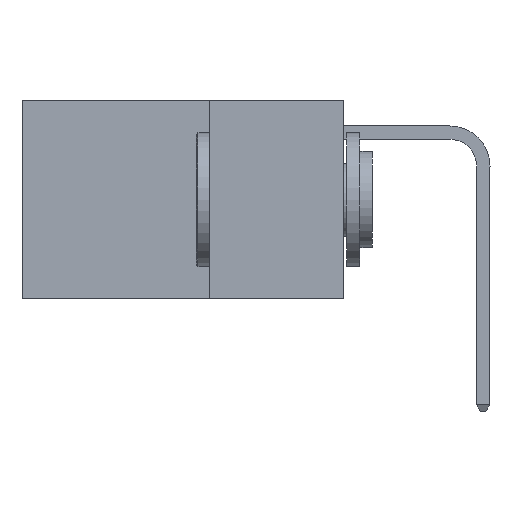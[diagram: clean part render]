
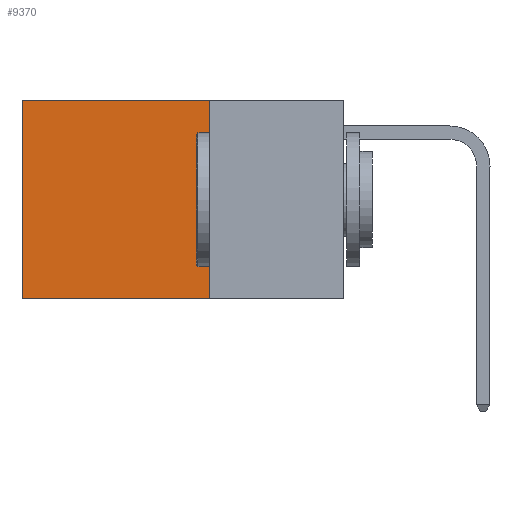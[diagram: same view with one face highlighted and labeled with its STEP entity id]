
A CAD part, left-side view. The second image highlights one B-rep face of the part: STEP entity #9370.
In plain terms, the highlighted planar face has unit normal (-1, 0, 0).
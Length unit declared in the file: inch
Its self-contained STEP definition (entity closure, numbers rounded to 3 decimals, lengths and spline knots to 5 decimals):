
#514 = EDGE_LOOP ( 'NONE', ( #15998, #1596, #9890, #17307 ) ) ;
#658 = CARTESIAN_POINT ( 'NONE',  ( 0.2625, 0.25, 0. ) ) ;
#696 = DIRECTION ( 'NONE',  ( 0., 0., -1. ) ) ;
#1596 = ORIENTED_EDGE ( 'NONE', *, *, #17029, .F. ) ;
#2420 = LINE ( 'NONE', #6323, #17493 ) ;
#3507 = DIRECTION ( 'NONE',  ( 0., 0., -1. ) ) ;
#3826 = VERTEX_POINT ( 'NONE', #658 ) ;
#3992 = VERTEX_POINT ( 'NONE', #5757 ) ;
#4047 = LINE ( 'NONE', #18514, #5840 ) ;
#4448 = EDGE_CURVE ( 'NONE', #9335, #3992, #13016, .T. ) ;
#4850 = EDGE_CURVE ( 'NONE', #3826, #9335, #2420, .T. ) ;
#5757 = CARTESIAN_POINT ( 'NONE',  ( 0.2625, 0.6, -0.37 ) ) ;
#5840 = VECTOR ( 'NONE', #3507, 39.37008 ) ;
#5875 = DIRECTION ( 'NONE',  ( 0., 0., -1. ) ) ;
#5886 = CARTESIAN_POINT ( 'NONE',  ( 0.2625, 0.6, 0. ) ) ;
#6323 = CARTESIAN_POINT ( 'NONE',  ( 0.2625, 0.25, 0. ) ) ;
#6891 = CARTESIAN_POINT ( 'NONE',  ( 0.2625, 0.25, -0.37 ) ) ;
#7074 = CARTESIAN_POINT ( 'NONE',  ( 0.2625, 0.25, -0.37 ) ) ;
#8128 = CARTESIAN_POINT ( 'NONE',  ( 0.2625, 0.6, 0. ) ) ;
#9335 = VERTEX_POINT ( 'NONE', #8128 ) ;
#9370 = ADVANCED_FACE ( 'NONE', ( #18680 ), #11130, .F. ) ;
#9466 = VECTOR ( 'NONE', #5875, 39.37008 ) ;
#9693 = DIRECTION ( 'NONE',  ( 1., 0., 0. ) ) ;
#9890 = ORIENTED_EDGE ( 'NONE', *, *, #16073, .F. ) ;
#10082 = VECTOR ( 'NONE', #19084, 39.37008 ) ;
#11130 = PLANE ( 'NONE',  #11276 ) ;
#11276 = AXIS2_PLACEMENT_3D ( 'NONE', #17231, #9693, #696 ) ;
#13016 = LINE ( 'NONE', #5886, #9466 ) ;
#13539 = DIRECTION ( 'NONE',  ( 0., 1., 0. ) ) ;
#14133 = LINE ( 'NONE', #7074, #10082 ) ;
#15998 = ORIENTED_EDGE ( 'NONE', *, *, #4448, .T. ) ;
#16073 = EDGE_CURVE ( 'NONE', #3826, #18242, #4047, .T. ) ;
#17029 = EDGE_CURVE ( 'NONE', #18242, #3992, #14133, .T. ) ;
#17231 = CARTESIAN_POINT ( 'NONE',  ( 0.2625, 0.25, 0. ) ) ;
#17307 = ORIENTED_EDGE ( 'NONE', *, *, #4850, .T. ) ;
#17493 = VECTOR ( 'NONE', #13539, 39.37008 ) ;
#18242 = VERTEX_POINT ( 'NONE', #6891 ) ;
#18514 = CARTESIAN_POINT ( 'NONE',  ( 0.2625, 0.25, 0. ) ) ;
#18680 = FACE_OUTER_BOUND ( 'NONE', #514, .T. ) ;
#19084 = DIRECTION ( 'NONE',  ( 0., 1., 0. ) ) ;
